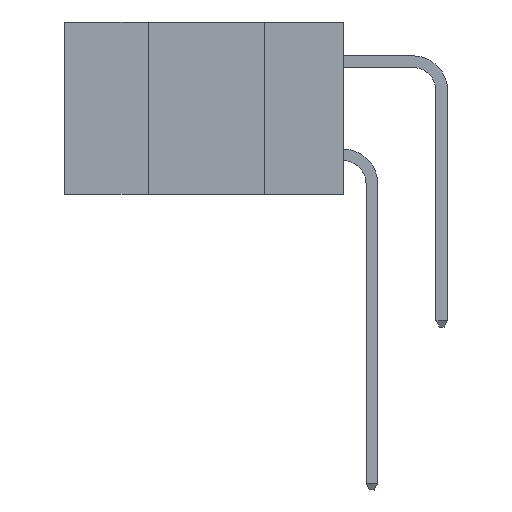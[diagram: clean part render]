
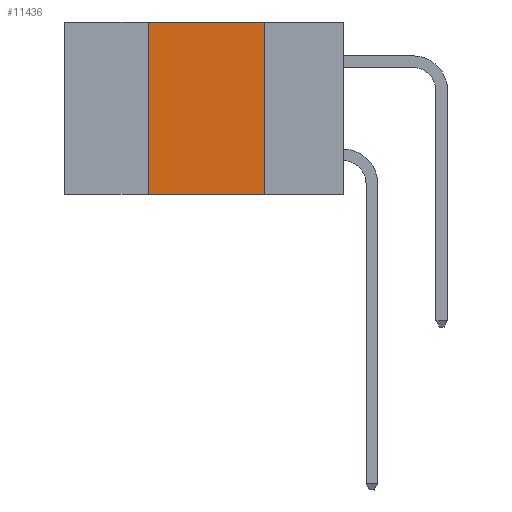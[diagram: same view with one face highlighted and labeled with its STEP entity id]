
A CAD part, left-side view. The second image highlights one B-rep face of the part: STEP entity #11436.
In plain terms, the highlighted planar face has unit normal (-1, 0, 0).
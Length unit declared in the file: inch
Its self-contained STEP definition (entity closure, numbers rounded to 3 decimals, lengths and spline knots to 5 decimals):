
#495 = LINE ( 'NONE', #21248, #26895 ) ;
#911 = CARTESIAN_POINT ( 'NONE',  ( 0., 0.6, 0. ) ) ;
#1289 = LINE ( 'NONE', #23090, #32890 ) ;
#1849 = EDGE_CURVE ( 'NONE', #16553, #27403, #7122, .T. ) ;
#5594 = DIRECTION ( 'NONE',  ( 0., 0., -1. ) ) ;
#6260 = DIRECTION ( 'NONE',  ( 1., 0., 0. ) ) ;
#7122 = LINE ( 'NONE', #11316, #13115 ) ;
#8798 = DIRECTION ( 'NONE',  ( 0., 0., -1. ) ) ;
#10639 = LINE ( 'NONE', #911, #16675 ) ;
#11316 = CARTESIAN_POINT ( 'NONE',  ( 0., 0.42, 0. ) ) ;
#11436 = ADVANCED_FACE ( 'NONE', ( #20910 ), #24036, .F. ) ;
#11823 = ORIENTED_EDGE ( 'NONE', *, *, #1849, .F. ) ;
#12074 = CARTESIAN_POINT ( 'NONE',  ( 0., 0.42, -0.37 ) ) ;
#12651 = EDGE_CURVE ( 'NONE', #27164, #30407, #495, .T. ) ;
#13115 = VECTOR ( 'NONE', #14128, 39.37008 ) ;
#13879 = CARTESIAN_POINT ( 'NONE',  ( 0., 0.17, 0. ) ) ;
#14128 = DIRECTION ( 'NONE',  ( 0., 0., 1. ) ) ;
#16325 = ORIENTED_EDGE ( 'NONE', *, *, #18477, .T. ) ;
#16553 = VERTEX_POINT ( 'NONE', #12074 ) ;
#16675 = VECTOR ( 'NONE', #31216, 39.37008 ) ;
#17423 = CARTESIAN_POINT ( 'NONE',  ( 0., 0.17, -0.37 ) ) ;
#18477 = EDGE_CURVE ( 'NONE', #16553, #30407, #1289, .T. ) ;
#20659 = ORIENTED_EDGE ( 'NONE', *, *, #12651, .F. ) ;
#20910 = FACE_OUTER_BOUND ( 'NONE', #25976, .T. ) ;
#21248 = CARTESIAN_POINT ( 'NONE',  ( 0., 0.17, 0. ) ) ;
#21695 = CARTESIAN_POINT ( 'NONE',  ( 0., 0.6, 0. ) ) ;
#23090 = CARTESIAN_POINT ( 'NONE',  ( 0., 0.6, -0.37 ) ) ;
#23306 = DIRECTION ( 'NONE',  ( 0., -1., 0. ) ) ;
#24036 = PLANE ( 'NONE',  #29960 ) ;
#25939 = CARTESIAN_POINT ( 'NONE',  ( 0., 0.42, 0. ) ) ;
#25976 = EDGE_LOOP ( 'NONE', ( #20659, #31266, #11823, #16325 ) ) ;
#26895 = VECTOR ( 'NONE', #5594, 39.37008 ) ;
#27164 = VERTEX_POINT ( 'NONE', #13879 ) ;
#27403 = VERTEX_POINT ( 'NONE', #25939 ) ;
#29960 = AXIS2_PLACEMENT_3D ( 'NONE', #21695, #6260, #8798 ) ;
#30407 = VERTEX_POINT ( 'NONE', #17423 ) ;
#31216 = DIRECTION ( 'NONE',  ( 0., -1., 0. ) ) ;
#31266 = ORIENTED_EDGE ( 'NONE', *, *, #32705, .F. ) ;
#32705 = EDGE_CURVE ( 'NONE', #27403, #27164, #10639, .T. ) ;
#32890 = VECTOR ( 'NONE', #23306, 39.37008 ) ;
